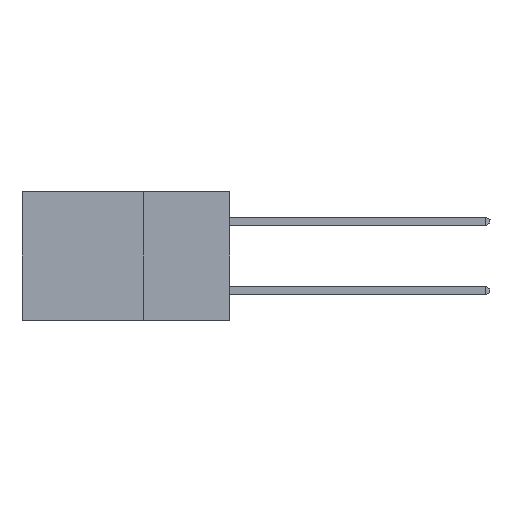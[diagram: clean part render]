
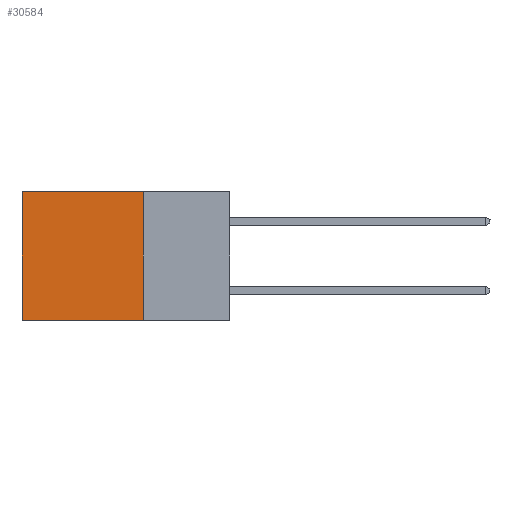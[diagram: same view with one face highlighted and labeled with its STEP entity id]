
A CAD part, left-side view. The second image highlights one B-rep face of the part: STEP entity #30584.
In plain terms, the highlighted planar face has unit normal (-1, 0, 0).
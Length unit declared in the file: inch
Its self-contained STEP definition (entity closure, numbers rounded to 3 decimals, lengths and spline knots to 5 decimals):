
#237 = CARTESIAN_POINT ( 'NONE',  ( 0.298, 0.6, -0.37 ) ) ;
#1616 = VECTOR ( 'NONE', #12406, 39.37008 ) ;
#2641 = CARTESIAN_POINT ( 'NONE',  ( 0.298, 0.25, 0. ) ) ;
#2654 = VERTEX_POINT ( 'NONE', #20293 ) ;
#3588 = LINE ( 'NONE', #2641, #21656 ) ;
#3780 = ORIENTED_EDGE ( 'NONE', *, *, #27757, .T. ) ;
#7455 = DIRECTION ( 'NONE',  ( 0., 1., 0. ) ) ;
#7567 = EDGE_LOOP ( 'NONE', ( #3780, #19449, #31368, #16929 ) ) ;
#7929 = VERTEX_POINT ( 'NONE', #32034 ) ;
#8138 = VERTEX_POINT ( 'NONE', #9647 ) ;
#9114 = VECTOR ( 'NONE', #7455, 39.37008 ) ;
#9156 = FACE_OUTER_BOUND ( 'NONE', #7567, .T. ) ;
#9647 = CARTESIAN_POINT ( 'NONE',  ( 0.298, 0.25, 0. ) ) ;
#10266 = CARTESIAN_POINT ( 'NONE',  ( 0.298, 0.25, -0.37 ) ) ;
#10768 = EDGE_CURVE ( 'NONE', #8138, #7929, #29581, .T. ) ;
#11187 = DIRECTION ( 'NONE',  ( 1., 0., 0. ) ) ;
#12406 = DIRECTION ( 'NONE',  ( 0., 0., -1. ) ) ;
#13873 = EDGE_CURVE ( 'NONE', #2654, #19788, #14969, .T. ) ;
#14969 = LINE ( 'NONE', #10266, #20952 ) ;
#15145 = EDGE_CURVE ( 'NONE', #8138, #2654, #3588, .T. ) ;
#15305 = LINE ( 'NONE', #32872, #1616 ) ;
#16929 = ORIENTED_EDGE ( 'NONE', *, *, #10768, .T. ) ;
#17610 = CARTESIAN_POINT ( 'NONE',  ( 0.298, 0.25, 0. ) ) ;
#18002 = DIRECTION ( 'NONE',  ( 0., 0., -1. ) ) ;
#19449 = ORIENTED_EDGE ( 'NONE', *, *, #13873, .F. ) ;
#19788 = VERTEX_POINT ( 'NONE', #237 ) ;
#20175 = AXIS2_PLACEMENT_3D ( 'NONE', #23942, #11187, #29136 ) ;
#20293 = CARTESIAN_POINT ( 'NONE',  ( 0.298, 0.25, -0.37 ) ) ;
#20952 = VECTOR ( 'NONE', #30770, 39.37008 ) ;
#21331 = PLANE ( 'NONE',  #20175 ) ;
#21656 = VECTOR ( 'NONE', #18002, 39.37008 ) ;
#23942 = CARTESIAN_POINT ( 'NONE',  ( 0.298, 0.25, 0. ) ) ;
#27757 = EDGE_CURVE ( 'NONE', #7929, #19788, #15305, .T. ) ;
#29136 = DIRECTION ( 'NONE',  ( 0., 0., -1. ) ) ;
#29581 = LINE ( 'NONE', #17610, #9114 ) ;
#30584 = ADVANCED_FACE ( 'NONE', ( #9156 ), #21331, .F. ) ;
#30770 = DIRECTION ( 'NONE',  ( 0., 1., 0. ) ) ;
#31368 = ORIENTED_EDGE ( 'NONE', *, *, #15145, .F. ) ;
#32034 = CARTESIAN_POINT ( 'NONE',  ( 0.298, 0.6, 0. ) ) ;
#32872 = CARTESIAN_POINT ( 'NONE',  ( 0.298, 0.6, 0. ) ) ;
